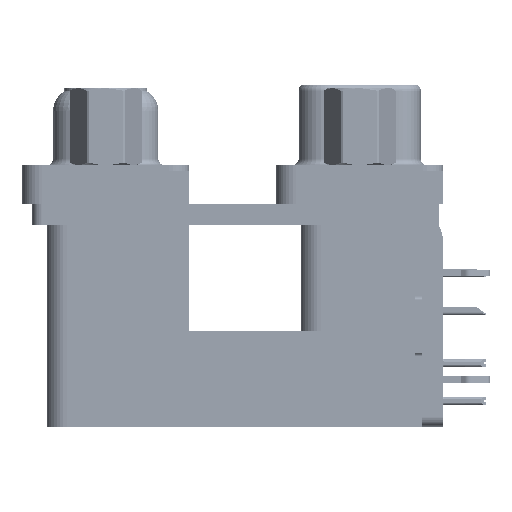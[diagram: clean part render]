
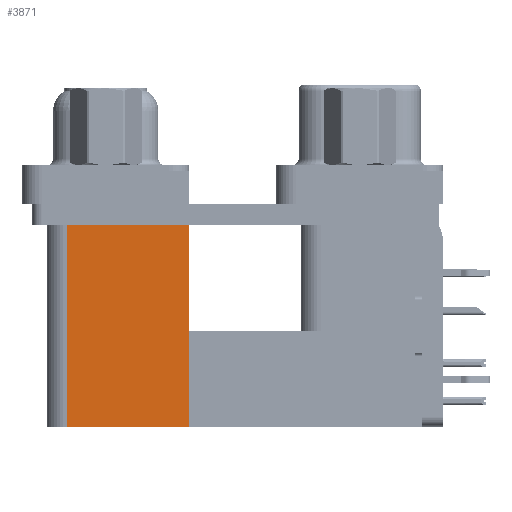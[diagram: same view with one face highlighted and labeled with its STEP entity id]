
A CAD part, left-side view. The second image highlights one B-rep face of the part: STEP entity #3871.
In plain terms, the highlighted planar face has unit normal (-1, 0, 0).
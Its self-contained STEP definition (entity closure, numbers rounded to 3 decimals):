
#834 = VECTOR ( 'NONE', #53570, 1000. ) ;
#3673 = VERTEX_POINT ( 'NONE', #4199 ) ;
#3871 = ADVANCED_FACE ( 'NONE', ( #30061 ), #58918, .F. ) ;
#4199 = CARTESIAN_POINT ( 'NONE',  ( 3.79, 12.775, -2.5 ) ) ;
#6338 = EDGE_CURVE ( 'NONE', #3673, #13560, #7812, .T. ) ;
#7210 = DIRECTION ( 'NONE',  ( 0., 1., 0. ) ) ;
#7567 = LINE ( 'NONE', #64976, #834 ) ;
#7812 = LINE ( 'NONE', #16485, #47106 ) ;
#9912 = DIRECTION ( 'NONE',  ( 0., 0., 1. ) ) ;
#11315 = EDGE_CURVE ( 'NONE', #71271, #13560, #28437, .T. ) ;
#11952 = CARTESIAN_POINT ( 'NONE',  ( 3.79, 21.975, -19.2 ) ) ;
#13560 = VERTEX_POINT ( 'NONE', #51803 ) ;
#16485 = CARTESIAN_POINT ( 'NONE',  ( 3.79, 12.775, -2.5 ) ) ;
#17156 = EDGE_CURVE ( 'NONE', #67168, #3673, #38101, .T. ) ;
#17456 = EDGE_CURVE ( 'NONE', #67168, #71271, #7567, .T. ) ;
#18636 = CARTESIAN_POINT ( 'NONE',  ( 3.79, 12.775, -19.2 ) ) ;
#27047 = CARTESIAN_POINT ( 'NONE',  ( 3.79, 12.775, -19.2 ) ) ;
#28437 = LINE ( 'NONE', #31998, #65972 ) ;
#28447 = ORIENTED_EDGE ( 'NONE', *, *, #17156, .T. ) ;
#30061 = FACE_OUTER_BOUND ( 'NONE', #41661, .T. ) ;
#31998 = CARTESIAN_POINT ( 'NONE',  ( 3.79, 21.975, -19.2 ) ) ;
#38101 = LINE ( 'NONE', #27047, #67602 ) ;
#39726 = DIRECTION ( 'NONE',  ( 0., 1., 0. ) ) ;
#41661 = EDGE_LOOP ( 'NONE', ( #60196, #64447, #57947, #28447 ) ) ;
#44511 = DIRECTION ( 'NONE',  ( 0., 0., 1. ) ) ;
#46405 = DIRECTION ( 'NONE',  ( 1., 0., 0. ) ) ;
#47106 = VECTOR ( 'NONE', #39726, 1000. ) ;
#51803 = CARTESIAN_POINT ( 'NONE',  ( 3.79, 21.975, -2.5 ) ) ;
#53570 = DIRECTION ( 'NONE',  ( 0., 1., 0. ) ) ;
#57947 = ORIENTED_EDGE ( 'NONE', *, *, #17456, .F. ) ;
#58918 = PLANE ( 'NONE',  #64210 ) ;
#60194 = CARTESIAN_POINT ( 'NONE',  ( 3.79, 12.775, -19.2 ) ) ;
#60196 = ORIENTED_EDGE ( 'NONE', *, *, #6338, .T. ) ;
#64210 = AXIS2_PLACEMENT_3D ( 'NONE', #18636, #46405, #7210 ) ;
#64447 = ORIENTED_EDGE ( 'NONE', *, *, #11315, .F. ) ;
#64976 = CARTESIAN_POINT ( 'NONE',  ( 3.79, 12.775, -19.2 ) ) ;
#65972 = VECTOR ( 'NONE', #44511, 1000. ) ;
#67168 = VERTEX_POINT ( 'NONE', #60194 ) ;
#67602 = VECTOR ( 'NONE', #9912, 1000. ) ;
#71271 = VERTEX_POINT ( 'NONE', #11952 ) ;
